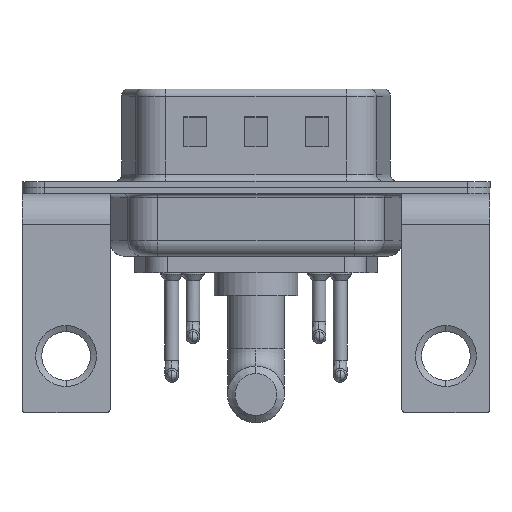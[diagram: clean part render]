
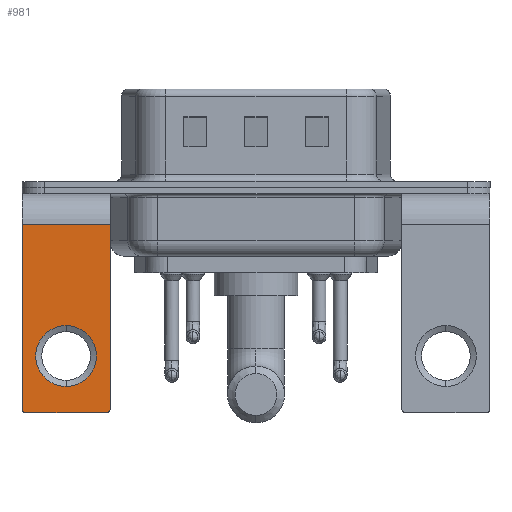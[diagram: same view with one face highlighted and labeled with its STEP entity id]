
A CAD part, front view. The second image highlights one B-rep face of the part: STEP entity #981.
In plain terms, the highlighted planar face has unit normal (0, -1, 0).
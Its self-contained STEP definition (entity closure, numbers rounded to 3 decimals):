
#59 = ORIENTED_EDGE ( 'NONE', *, *, #6415, .T. ) ;
#520 = CARTESIAN_POINT ( 'NONE',  ( 0., -6.25, -11.07 ) ) ;
#609 = EDGE_CURVE ( 'NONE', #9989, #4179, #3082, .T. ) ;
#661 = ORIENTED_EDGE ( 'NONE', *, *, #11235, .T. ) ;
#887 = CIRCLE ( 'NONE', #10429, 0.25 ) ;
#981 = ADVANCED_FACE ( 'NONE', ( #9235, #13916 ), #7771, .F. ) ;
#1180 = CARTESIAN_POINT ( 'NONE',  ( -2.9, -6.25, -2.4 ) ) ;
#1255 = CARTESIAN_POINT ( 'NONE',  ( 0., -6.25, -13.07 ) ) ;
#2535 = CIRCLE ( 'NONE', #5475, 0.25 ) ;
#3082 = LINE ( 'NONE', #8305, #9960 ) ;
#3102 = VERTEX_POINT ( 'NONE', #19028 ) ;
#3253 = CARTESIAN_POINT ( 'NONE',  ( 2.9, -6.25, -2.4 ) ) ;
#3608 = CARTESIAN_POINT ( 'NONE',  ( 0., -6.25, -11.07 ) ) ;
#3935 = EDGE_LOOP ( 'NONE', ( #59, #11519 ) ) ;
#4040 = EDGE_CURVE ( 'NONE', #10101, #3102, #9403, .T. ) ;
#4179 = VERTEX_POINT ( 'NONE', #19624 ) ;
#4361 = VECTOR ( 'NONE', #19557, 1000. ) ;
#5246 = VERTEX_POINT ( 'NONE', #1255 ) ;
#5388 = DIRECTION ( 'NONE',  ( 0., 0., 1. ) ) ;
#5443 = DIRECTION ( 'NONE',  ( 0., 1., 0. ) ) ;
#5475 = AXIS2_PLACEMENT_3D ( 'NONE', #11575, #19446, #5388 ) ;
#5911 = LINE ( 'NONE', #1180, #17544 ) ;
#6036 = AXIS2_PLACEMENT_3D ( 'NONE', #3608, #14167, #17364 ) ;
#6415 = EDGE_CURVE ( 'NONE', #5246, #14511, #13049, .T. ) ;
#6437 = VECTOR ( 'NONE', #12455, 1000. ) ;
#7353 = LINE ( 'NONE', #11676, #4361 ) ;
#7362 = CIRCLE ( 'NONE', #6036, 2. ) ;
#7771 = PLANE ( 'NONE',  #10016 ) ;
#7831 = ORIENTED_EDGE ( 'NONE', *, *, #13861, .T. ) ;
#7877 = CARTESIAN_POINT ( 'NONE',  ( 2.9, -6.25, -2.4 ) ) ;
#8305 = CARTESIAN_POINT ( 'NONE',  ( 2.9, -6.25, -14.8 ) ) ;
#8789 = CARTESIAN_POINT ( 'NONE',  ( -2.9, -6.25, -2.4 ) ) ;
#9167 = DIRECTION ( 'NONE',  ( 0., -1., 0. ) ) ;
#9235 = FACE_BOUND ( 'NONE', #3935, .T. ) ;
#9403 = LINE ( 'NONE', #19102, #6437 ) ;
#9762 = DIRECTION ( 'NONE',  ( -1., 0., 0. ) ) ;
#9960 = VECTOR ( 'NONE', #9762, 1000. ) ;
#9989 = VERTEX_POINT ( 'NONE', #16629 ) ;
#10016 = AXIS2_PLACEMENT_3D ( 'NONE', #7877, #14024, #15456 ) ;
#10101 = VERTEX_POINT ( 'NONE', #3253 ) ;
#10104 = DIRECTION ( 'NONE',  ( 0., 0., 1. ) ) ;
#10429 = AXIS2_PLACEMENT_3D ( 'NONE', #18671, #9167, #15479 ) ;
#11021 = ORIENTED_EDGE ( 'NONE', *, *, #609, .F. ) ;
#11235 = EDGE_CURVE ( 'NONE', #14915, #4179, #887, .T. ) ;
#11519 = ORIENTED_EDGE ( 'NONE', *, *, #14538, .T. ) ;
#11575 = CARTESIAN_POINT ( 'NONE',  ( 2.65, -6.25, -14.55 ) ) ;
#11676 = CARTESIAN_POINT ( 'NONE',  ( 2.9, -6.25, -2.4 ) ) ;
#11817 = EDGE_LOOP ( 'NONE', ( #13435, #661, #11021, #14176, #17519, #7831 ) ) ;
#12080 = DIRECTION ( 'NONE',  ( 0., 0., -1. ) ) ;
#12455 = DIRECTION ( 'NONE',  ( 0., 0., -1. ) ) ;
#13049 = CIRCLE ( 'NONE', #15983, 2. ) ;
#13435 = ORIENTED_EDGE ( 'NONE', *, *, #15993, .T. ) ;
#13861 = EDGE_CURVE ( 'NONE', #10101, #16354, #7353, .T. ) ;
#13916 = FACE_OUTER_BOUND ( 'NONE', #11817, .T. ) ;
#14024 = DIRECTION ( 'NONE',  ( 0., 1., 0. ) ) ;
#14167 = DIRECTION ( 'NONE',  ( 0., 1., 0. ) ) ;
#14176 = ORIENTED_EDGE ( 'NONE', *, *, #17044, .T. ) ;
#14511 = VERTEX_POINT ( 'NONE', #18797 ) ;
#14538 = EDGE_CURVE ( 'NONE', #14511, #5246, #7362, .T. ) ;
#14915 = VERTEX_POINT ( 'NONE', #16153 ) ;
#15456 = DIRECTION ( 'NONE',  ( 0., 0., 1. ) ) ;
#15479 = DIRECTION ( 'NONE',  ( 0., 0., 1. ) ) ;
#15983 = AXIS2_PLACEMENT_3D ( 'NONE', #520, #5443, #10104 ) ;
#15993 = EDGE_CURVE ( 'NONE', #16354, #14915, #5911, .T. ) ;
#16153 = CARTESIAN_POINT ( 'NONE',  ( -2.9, -6.25, -14.55 ) ) ;
#16354 = VERTEX_POINT ( 'NONE', #8789 ) ;
#16629 = CARTESIAN_POINT ( 'NONE',  ( 2.65, -6.25, -14.8 ) ) ;
#17044 = EDGE_CURVE ( 'NONE', #9989, #3102, #2535, .T. ) ;
#17364 = DIRECTION ( 'NONE',  ( 0., 0., 1. ) ) ;
#17519 = ORIENTED_EDGE ( 'NONE', *, *, #4040, .F. ) ;
#17544 = VECTOR ( 'NONE', #12080, 1000. ) ;
#18671 = CARTESIAN_POINT ( 'NONE',  ( -2.65, -6.25, -14.55 ) ) ;
#18797 = CARTESIAN_POINT ( 'NONE',  ( 0., -6.25, -9.07 ) ) ;
#19028 = CARTESIAN_POINT ( 'NONE',  ( 2.9, -6.25, -14.55 ) ) ;
#19102 = CARTESIAN_POINT ( 'NONE',  ( 2.9, -6.25, -2.4 ) ) ;
#19446 = DIRECTION ( 'NONE',  ( 0., -1., 0. ) ) ;
#19557 = DIRECTION ( 'NONE',  ( -1., 0., 0. ) ) ;
#19624 = CARTESIAN_POINT ( 'NONE',  ( -2.65, -6.25, -14.8 ) ) ;
